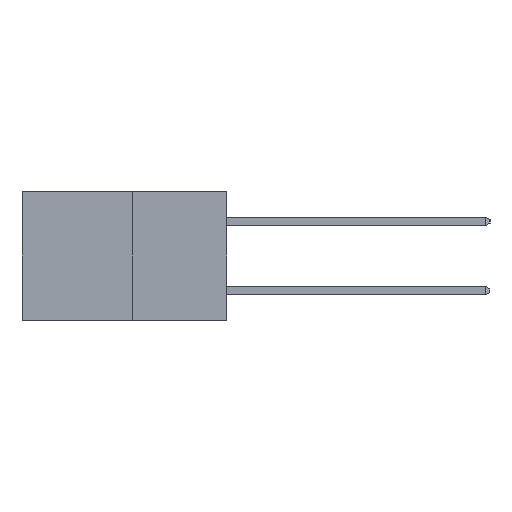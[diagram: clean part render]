
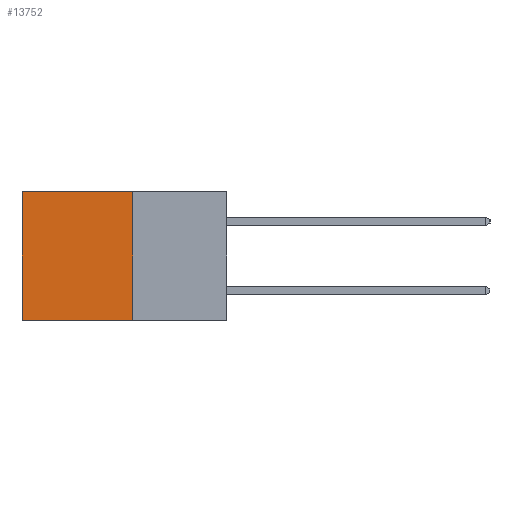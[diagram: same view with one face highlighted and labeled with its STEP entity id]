
A CAD part, left-side view. The second image highlights one B-rep face of the part: STEP entity #13752.
In plain terms, the highlighted planar face has unit normal (-1, 0, 0).
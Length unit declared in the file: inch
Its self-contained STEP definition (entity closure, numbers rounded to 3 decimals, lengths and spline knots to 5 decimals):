
#487 = DIRECTION ( 'NONE',  ( 0., 1., 0. ) ) ;
#655 = VECTOR ( 'NONE', #487, 39.37008 ) ;
#1326 = ORIENTED_EDGE ( 'NONE', *, *, #7420, .T. ) ;
#1662 = CARTESIAN_POINT ( 'NONE',  ( 0.277, 0.27, -0.37 ) ) ;
#1754 = ORIENTED_EDGE ( 'NONE', *, *, #6525, .T. ) ;
#2035 = VECTOR ( 'NONE', #4665, 39.37008 ) ;
#2657 = LINE ( 'NONE', #14833, #3111 ) ;
#3069 = DIRECTION ( 'NONE',  ( 0., 0., -1. ) ) ;
#3080 = VERTEX_POINT ( 'NONE', #10839 ) ;
#3111 = VECTOR ( 'NONE', #5887, 39.37008 ) ;
#3140 = VERTEX_POINT ( 'NONE', #15225 ) ;
#4547 = FACE_OUTER_BOUND ( 'NONE', #10913, .T. ) ;
#4665 = DIRECTION ( 'NONE',  ( 0., 0., -1. ) ) ;
#5255 = DIRECTION ( 'NONE',  ( 0., 1., 0. ) ) ;
#5858 = EDGE_CURVE ( 'NONE', #10995, #3080, #9034, .T. ) ;
#5887 = DIRECTION ( 'NONE',  ( 0., 0., -1. ) ) ;
#6525 = EDGE_CURVE ( 'NONE', #3140, #7366, #2657, .T. ) ;
#6983 = PLANE ( 'NONE',  #14967 ) ;
#7239 = CARTESIAN_POINT ( 'NONE',  ( 0.277, 0.27, -0.37 ) ) ;
#7259 = ORIENTED_EDGE ( 'NONE', *, *, #12656, .F. ) ;
#7366 = VERTEX_POINT ( 'NONE', #10309 ) ;
#7420 = EDGE_CURVE ( 'NONE', #10995, #3140, #13779, .T. ) ;
#8601 = LINE ( 'NONE', #7239, #655 ) ;
#9034 = LINE ( 'NONE', #11100, #2035 ) ;
#9130 = CARTESIAN_POINT ( 'NONE',  ( 0.277, 0.27, 0. ) ) ;
#9976 = VECTOR ( 'NONE', #5255, 39.37008 ) ;
#10309 = CARTESIAN_POINT ( 'NONE',  ( 0.277, 0.59, -0.37 ) ) ;
#10839 = CARTESIAN_POINT ( 'NONE',  ( 0.277, 0.27, -0.37 ) ) ;
#10850 = DIRECTION ( 'NONE',  ( 1., 0., 0. ) ) ;
#10913 = EDGE_LOOP ( 'NONE', ( #1754, #7259, #11956, #1326 ) ) ;
#10995 = VERTEX_POINT ( 'NONE', #15030 ) ;
#11100 = CARTESIAN_POINT ( 'NONE',  ( 0.277, 0.27, -0.37 ) ) ;
#11956 = ORIENTED_EDGE ( 'NONE', *, *, #5858, .F. ) ;
#12656 = EDGE_CURVE ( 'NONE', #3080, #7366, #8601, .T. ) ;
#13752 = ADVANCED_FACE ( 'NONE', ( #4547 ), #6983, .F. ) ;
#13779 = LINE ( 'NONE', #9130, #9976 ) ;
#14833 = CARTESIAN_POINT ( 'NONE',  ( 0.277, 0.59, -0.37 ) ) ;
#14967 = AXIS2_PLACEMENT_3D ( 'NONE', #1662, #10850, #3069 ) ;
#15030 = CARTESIAN_POINT ( 'NONE',  ( 0.277, 0.27, 0. ) ) ;
#15225 = CARTESIAN_POINT ( 'NONE',  ( 0.277, 0.59, 0. ) ) ;
